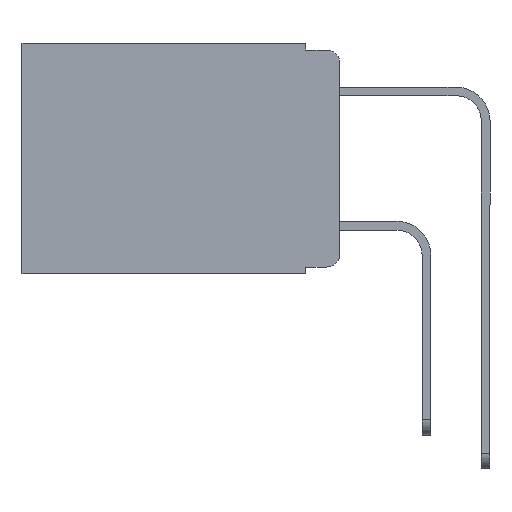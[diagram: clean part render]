
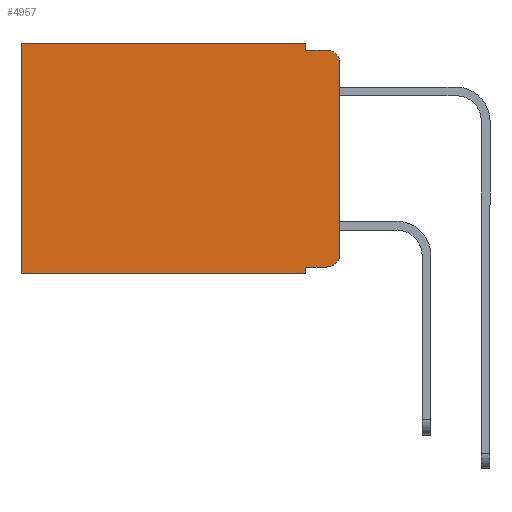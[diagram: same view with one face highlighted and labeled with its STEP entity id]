
A CAD part, left-side view. The second image highlights one B-rep face of the part: STEP entity #4957.
In plain terms, the highlighted planar face has unit normal (-1, 0, 0).
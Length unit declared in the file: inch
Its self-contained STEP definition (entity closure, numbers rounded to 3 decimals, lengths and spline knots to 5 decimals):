
#115 = EDGE_CURVE ( 'NONE', #765, #3229, #1777, .T. ) ;
#343 = DIRECTION ( 'NONE',  ( 0., 0., -1. ) ) ;
#765 = VERTEX_POINT ( 'NONE', #11937 ) ;
#866 = VECTOR ( 'NONE', #343, 39.37008 ) ;
#1053 = VECTOR ( 'NONE', #6357, 39.37008 ) ;
#1122 = DIRECTION ( 'NONE',  ( 0., 0., -1. ) ) ;
#1302 = VERTEX_POINT ( 'NONE', #10569 ) ;
#1324 = PLANE ( 'NONE',  #7913 ) ;
#1499 = VERTEX_POINT ( 'NONE', #8050 ) ;
#1652 = EDGE_CURVE ( 'NONE', #10318, #9113, #11478, .T. ) ;
#1729 = VECTOR ( 'NONE', #11433, 39.37008 ) ;
#1777 = LINE ( 'NONE', #7598, #4051 ) ;
#1887 = CARTESIAN_POINT ( 'NONE',  ( 0.298, 0., 0. ) ) ;
#1947 = ORIENTED_EDGE ( 'NONE', *, *, #8034, .T. ) ;
#2063 = CARTESIAN_POINT ( 'NONE',  ( 0.298, 0.473, 0. ) ) ;
#2415 = VERTEX_POINT ( 'NONE', #5302 ) ;
#2426 = DIRECTION ( 'NONE',  ( 0., 1., 0. ) ) ;
#2515 = LINE ( 'NONE', #3150, #12193 ) ;
#2898 = CARTESIAN_POINT ( 'NONE',  ( 0.298, 0.02, -0.313 ) ) ;
#2983 = LINE ( 'NONE', #9590, #3297 ) ;
#3098 = CARTESIAN_POINT ( 'NONE',  ( 0.298, 0.02, -0.01 ) ) ;
#3150 = CARTESIAN_POINT ( 'NONE',  ( 0.298, 0.051, 0. ) ) ;
#3224 = EDGE_CURVE ( 'NONE', #9113, #8390, #12127, .T. ) ;
#3229 = VERTEX_POINT ( 'NONE', #2063 ) ;
#3233 = DIRECTION ( 'NONE',  ( 0., -1., 0. ) ) ;
#3242 = DIRECTION ( 'NONE',  ( 0., 0., -1. ) ) ;
#3251 = DIRECTION ( 'NONE',  ( -1., 0., 0. ) ) ;
#3297 = VECTOR ( 'NONE', #7984, 39.37008 ) ;
#3387 = VECTOR ( 'NONE', #3233, 39.37008 ) ;
#3529 = EDGE_CURVE ( 'NONE', #765, #1499, #3628, .T. ) ;
#3628 = LINE ( 'NONE', #10334, #1053 ) ;
#4051 = VECTOR ( 'NONE', #2426, 39.37008 ) ;
#4149 = DIRECTION ( 'NONE',  ( 0., 1., 0. ) ) ;
#4396 = ORIENTED_EDGE ( 'NONE', *, *, #5966, .F. ) ;
#4420 = ORIENTED_EDGE ( 'NONE', *, *, #1652, .T. ) ;
#4509 = CARTESIAN_POINT ( 'NONE',  ( 0.298, 0., -0.313 ) ) ;
#4516 = VECTOR ( 'NONE', #4149, 39.37008 ) ;
#4743 = AXIS2_PLACEMENT_3D ( 'NONE', #7357, #6409, #1122 ) ;
#4957 = ADVANCED_FACE ( 'NONE', ( #5149 ), #1324, .F. ) ;
#5149 = FACE_OUTER_BOUND ( 'NONE', #10277, .T. ) ;
#5302 = CARTESIAN_POINT ( 'NONE',  ( 0.298, 0.051, -0.343 ) ) ;
#5594 = EDGE_CURVE ( 'NONE', #3229, #1302, #2983, .T. ) ;
#5635 = CARTESIAN_POINT ( 'NONE',  ( 0.298, 0.051, -0.333 ) ) ;
#5966 = EDGE_CURVE ( 'NONE', #2415, #1302, #11677, .T. ) ;
#6038 = LINE ( 'NONE', #1887, #866 ) ;
#6357 = DIRECTION ( 'NONE',  ( 0., 0., -1. ) ) ;
#6409 = DIRECTION ( 'NONE',  ( -1., 0., 0. ) ) ;
#6414 = VERTEX_POINT ( 'NONE', #3098 ) ;
#6492 = DIRECTION ( 'NONE',  ( 0., 0., -1. ) ) ;
#6742 = EDGE_CURVE ( 'NONE', #10318, #2415, #2515, .T. ) ;
#6783 = CARTESIAN_POINT ( 'NONE',  ( 0.298, 0., -0.03 ) ) ;
#7357 = CARTESIAN_POINT ( 'NONE',  ( 0.298, 0.02, -0.03 ) ) ;
#7598 = CARTESIAN_POINT ( 'NONE',  ( 0.298, 0., 0. ) ) ;
#7913 = AXIS2_PLACEMENT_3D ( 'NONE', #9457, #10698, #10850 ) ;
#7954 = ORIENTED_EDGE ( 'NONE', *, *, #3529, .F. ) ;
#7971 = ORIENTED_EDGE ( 'NONE', *, *, #9623, .F. ) ;
#7984 = DIRECTION ( 'NONE',  ( 0., 0., -1. ) ) ;
#8034 = EDGE_CURVE ( 'NONE', #10811, #6414, #9028, .T. ) ;
#8050 = CARTESIAN_POINT ( 'NONE',  ( 0.298, 0.051, -0.01 ) ) ;
#8196 = ORIENTED_EDGE ( 'NONE', *, *, #3224, .T. ) ;
#8262 = ORIENTED_EDGE ( 'NONE', *, *, #6742, .F. ) ;
#8390 = VERTEX_POINT ( 'NONE', #4509 ) ;
#8471 = LINE ( 'NONE', #10776, #3387 ) ;
#9028 = CIRCLE ( 'NONE', #4743, 0.02 ) ;
#9113 = VERTEX_POINT ( 'NONE', #10663 ) ;
#9284 = AXIS2_PLACEMENT_3D ( 'NONE', #2898, #3251, #3242 ) ;
#9457 = CARTESIAN_POINT ( 'NONE',  ( 0.298, 0., 0. ) ) ;
#9517 = CARTESIAN_POINT ( 'NONE',  ( 0.298, 0.051, -0.333 ) ) ;
#9590 = CARTESIAN_POINT ( 'NONE',  ( 0.298, 0.473, 0. ) ) ;
#9623 = EDGE_CURVE ( 'NONE', #10811, #8390, #6038, .T. ) ;
#10092 = ORIENTED_EDGE ( 'NONE', *, *, #5594, .T. ) ;
#10148 = CARTESIAN_POINT ( 'NONE',  ( 0.298, 0., -0.343 ) ) ;
#10277 = EDGE_LOOP ( 'NONE', ( #7971, #1947, #12236, #7954, #10682, #10092, #4396, #8262, #4420, #8196 ) ) ;
#10318 = VERTEX_POINT ( 'NONE', #5635 ) ;
#10334 = CARTESIAN_POINT ( 'NONE',  ( 0.298, 0.051, 0. ) ) ;
#10569 = CARTESIAN_POINT ( 'NONE',  ( 0.298, 0.473, -0.343 ) ) ;
#10663 = CARTESIAN_POINT ( 'NONE',  ( 0.298, 0.02, -0.333 ) ) ;
#10682 = ORIENTED_EDGE ( 'NONE', *, *, #115, .T. ) ;
#10698 = DIRECTION ( 'NONE',  ( 1., 0., 0. ) ) ;
#10776 = CARTESIAN_POINT ( 'NONE',  ( 0.298, 0.051, -0.01 ) ) ;
#10811 = VERTEX_POINT ( 'NONE', #6783 ) ;
#10850 = DIRECTION ( 'NONE',  ( 0., 0., -1. ) ) ;
#11433 = DIRECTION ( 'NONE',  ( 0., -1., 0. ) ) ;
#11478 = LINE ( 'NONE', #9517, #1729 ) ;
#11677 = LINE ( 'NONE', #10148, #4516 ) ;
#11937 = CARTESIAN_POINT ( 'NONE',  ( 0.298, 0.051, 0. ) ) ;
#12088 = EDGE_CURVE ( 'NONE', #1499, #6414, #8471, .T. ) ;
#12127 = CIRCLE ( 'NONE', #9284, 0.02 ) ;
#12193 = VECTOR ( 'NONE', #6492, 39.37008 ) ;
#12236 = ORIENTED_EDGE ( 'NONE', *, *, #12088, .F. ) ;
